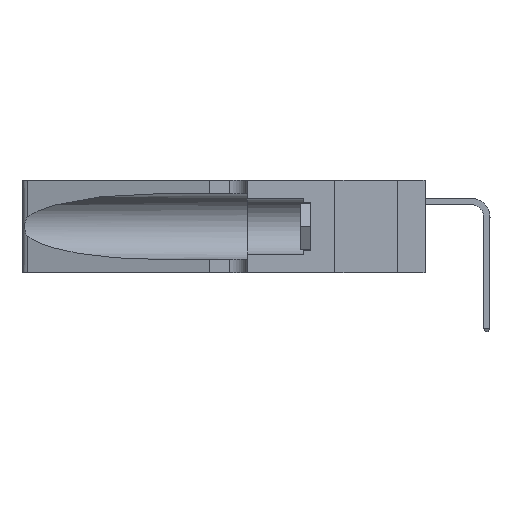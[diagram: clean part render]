
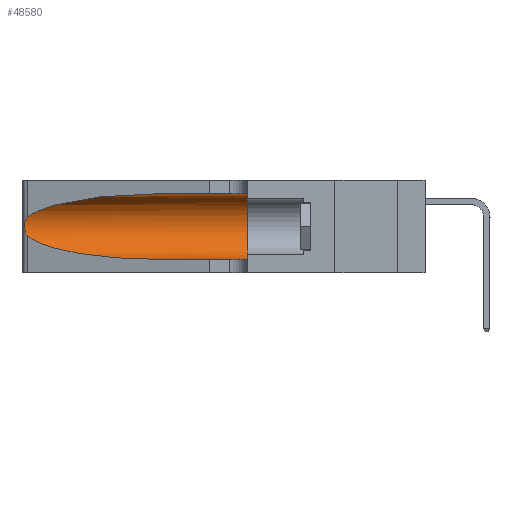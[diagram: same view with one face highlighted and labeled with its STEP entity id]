
A CAD part, left-side view. The second image highlights one B-rep face of the part: STEP entity #48580.
In plain terms, the highlighted cylindrical face has radius 3.308 mm (diameter 6.617 mm), a partial arc.
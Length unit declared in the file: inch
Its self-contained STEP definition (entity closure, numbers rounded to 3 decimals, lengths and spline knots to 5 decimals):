
#580 = EDGE_CURVE ( 'NONE', #8958, #18083, #6610, .T. ) ;
#670 = CARTESIAN_POINT ( 'NONE',  ( 0.1305, 1.61858, 0.185 ) ) ;
#961 =( BOUNDED_CURVE ( )  B_SPLINE_CURVE ( 3, ( #18352, #45907, #49839, #26340 ),
 .UNSPECIFIED., .F., .F. ) 
 B_SPLINE_CURVE_WITH_KNOTS ( ( 4, 4 ),
 ( 1.5708, 2.84003 ),
 .UNSPECIFIED. ) 
 CURVE ( )  GEOMETRIC_REPRESENTATION_ITEM ( )  RATIONAL_B_SPLINE_CURVE ( ( 1., 0.87, 0.87, 1. ) ) 
 REPRESENTATION_ITEM ( '' )  );
#1910 = ORIENTED_EDGE ( 'NONE', *, *, #4450, .F. ) ;
#3669 = FACE_OUTER_BOUND ( 'NONE', #18186, .T. ) ;
#3738 = CARTESIAN_POINT ( 'NONE',  ( 0.26017, 1.23833, 0.17102 ) ) ;
#4008 = CIRCLE ( 'NONE', #46564, 0.13025 ) ;
#4450 = EDGE_CURVE ( 'NONE', #8155, #47594, #37714, .T. ) ;
#4682 = ORIENTED_EDGE ( 'NONE', *, *, #50196, .T. ) ;
#5480 = AXIS2_PLACEMENT_3D ( 'NONE', #670, #16592, #28592 ) ;
#6610 = B_SPLINE_CURVE_WITH_KNOTS ( 'NONE', 3,
 ( #43254, #31450, #39309, #19701, #47174, #23704, #51121, #27657, #3738, #31633, #7744, #35536, #11764, #39473 ),
 .UNSPECIFIED., .F., .F.,
 ( 4, 2, 2, 2, 2, 2, 4 ),
 ( 0., 0.00027, 0.00053, 0.00107, 0.0016, 0.00187, 0.00214 ),
 .UNSPECIFIED. ) ;
#7744 = CARTESIAN_POINT ( 'NONE',  ( 0.25789, 1.23486, 0.15765 ) ) ;
#7837 = VERTEX_POINT ( 'NONE', #42250 ) ;
#8155 = VERTEX_POINT ( 'NONE', #17759 ) ;
#8160 = CARTESIAN_POINT ( 'NONE',  ( 0.1305, 0.72297, 0.05475 ) ) ;
#8232 = ORIENTED_EDGE ( 'NONE', *, *, #27090, .T. ) ;
#8958 = VERTEX_POINT ( 'NONE', #38202 ) ;
#10351 = LINE ( 'NONE', #13061, #18533 ) ;
#11764 = CARTESIAN_POINT ( 'NONE',  ( 0.25555, 1.22993, 0.14849 ) ) ;
#13061 = CARTESIAN_POINT ( 'NONE',  ( 0.1305, 1.61858, 0.05475 ) ) ;
#14310 = EDGE_CURVE ( 'NONE', #47594, #7837, #4008, .T. ) ;
#14456 = CARTESIAN_POINT ( 'NONE',  ( 0.1305, 0.35, 0.185 ) ) ;
#16592 = DIRECTION ( 'NONE',  ( 0., -1., 0. ) ) ;
#17318 = EDGE_CURVE ( 'NONE', #8155, #8958, #961, .T. ) ;
#17759 = CARTESIAN_POINT ( 'NONE',  ( 0.1305, 0.72297, 0.31525 ) ) ;
#18083 = VERTEX_POINT ( 'NONE', #38610 ) ;
#18186 = EDGE_LOOP ( 'NONE', ( #34657, #50207, #4682, #8232, #22065, #1910 ) ) ;
#18352 = CARTESIAN_POINT ( 'NONE',  ( 0.1305, 0.72297, 0.31525 ) ) ;
#18499 = DIRECTION ( 'NONE',  ( 0., 0., 1. ) ) ;
#18533 = VECTOR ( 'NONE', #21148, 39.37008 ) ;
#19671 = CARTESIAN_POINT ( 'NONE',  ( 0.1305, 0.72297, 0.05475 ) ) ;
#19701 = CARTESIAN_POINT ( 'NONE',  ( 0.25787, 1.23484, 0.2124 ) ) ;
#21148 = DIRECTION ( 'NONE',  ( 0., -1., 0. ) ) ;
#22065 = ORIENTED_EDGE ( 'NONE', *, *, #14310, .F. ) ;
#23411 = CARTESIAN_POINT ( 'NONE',  ( 0.1305, 1.61858, 0.31525 ) ) ;
#23704 = CARTESIAN_POINT ( 'NONE',  ( 0.26018, 1.23835, 0.19895 ) ) ;
#26340 = CARTESIAN_POINT ( 'NONE',  ( 0.25487, 1.22718, 0.22369 ) ) ;
#26938 = CARTESIAN_POINT ( 'NONE',  ( 0.1305, 0.35, 0.31525 ) ) ;
#27090 = EDGE_CURVE ( 'NONE', #30538, #7837, #10351, .T. ) ;
#27305 = VECTOR ( 'NONE', #31346, 39.37008 ) ;
#27657 = CARTESIAN_POINT ( 'NONE',  ( 0.26075, 1.23896, 0.178 ) ) ;
#28592 = DIRECTION ( 'NONE',  ( 0., 0., -1. ) ) ;
#30538 = VERTEX_POINT ( 'NONE', #8160 ) ;
#31346 = DIRECTION ( 'NONE',  ( 0., -1., 0. ) ) ;
#31450 = CARTESIAN_POINT ( 'NONE',  ( 0.25555, 1.22994, 0.2215 ) ) ;
#31633 = CARTESIAN_POINT ( 'NONE',  ( 0.25856, 1.23593, 0.16098 ) ) ;
#34180 = CYLINDRICAL_SURFACE ( 'NONE', #5480, 0.13025 ) ;
#34262 =( BOUNDED_CURVE ( )  B_SPLINE_CURVE ( 3, ( #35340, #50917, #43215, #19671 ),
 .UNSPECIFIED., .F., .F. ) 
 B_SPLINE_CURVE_WITH_KNOTS ( ( 4, 4 ),
 ( 3.44316, 4.71239 ),
 .UNSPECIFIED. ) 
 CURVE ( )  GEOMETRIC_REPRESENTATION_ITEM ( )  RATIONAL_B_SPLINE_CURVE ( ( 1., 0.87, 0.87, 1. ) ) 
 REPRESENTATION_ITEM ( '' )  );
#34657 = ORIENTED_EDGE ( 'NONE', *, *, #17318, .T. ) ;
#35340 = CARTESIAN_POINT ( 'NONE',  ( 0.25487, 1.22718, 0.14631 ) ) ;
#35536 = CARTESIAN_POINT ( 'NONE',  ( 0.25639, 1.23186, 0.15144 ) ) ;
#37714 = LINE ( 'NONE', #23411, #27305 ) ;
#38202 = CARTESIAN_POINT ( 'NONE',  ( 0.25487, 1.22718, 0.22369 ) ) ;
#38610 = CARTESIAN_POINT ( 'NONE',  ( 0.25487, 1.22718, 0.14631 ) ) ;
#39309 = CARTESIAN_POINT ( 'NONE',  ( 0.25639, 1.23184, 0.21858 ) ) ;
#39473 = CARTESIAN_POINT ( 'NONE',  ( 0.25487, 1.22718, 0.14631 ) ) ;
#42126 = DIRECTION ( 'NONE',  ( 0., 1., 0. ) ) ;
#42250 = CARTESIAN_POINT ( 'NONE',  ( 0.1305, 0.35, 0.05475 ) ) ;
#43215 = CARTESIAN_POINT ( 'NONE',  ( 0.18966, 0.96281, 0.05475 ) ) ;
#43254 = CARTESIAN_POINT ( 'NONE',  ( 0.25487, 1.22718, 0.22369 ) ) ;
#45907 = CARTESIAN_POINT ( 'NONE',  ( 0.18966, 0.96281, 0.31525 ) ) ;
#46564 = AXIS2_PLACEMENT_3D ( 'NONE', #14456, #42126, #18499 ) ;
#47174 = CARTESIAN_POINT ( 'NONE',  ( 0.25854, 1.2359, 0.20912 ) ) ;
#47594 = VERTEX_POINT ( 'NONE', #26938 ) ;
#48580 = ADVANCED_FACE ( 'NONE', ( #3669 ), #34180, .F. ) ;
#49839 = CARTESIAN_POINT ( 'NONE',  ( 0.2373, 1.15595, 0.28018 ) ) ;
#50196 = EDGE_CURVE ( 'NONE', #18083, #30538, #34262, .T. ) ;
#50207 = ORIENTED_EDGE ( 'NONE', *, *, #580, .T. ) ;
#50917 = CARTESIAN_POINT ( 'NONE',  ( 0.2373, 1.15595, 0.08982 ) ) ;
#51121 = CARTESIAN_POINT ( 'NONE',  ( 0.26075, 1.23896, 0.19203 ) ) ;
